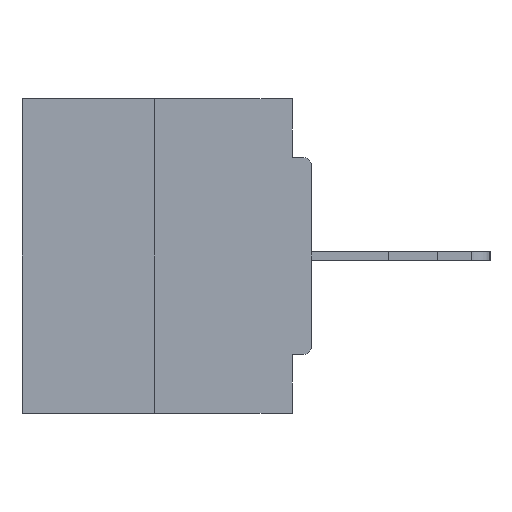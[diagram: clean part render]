
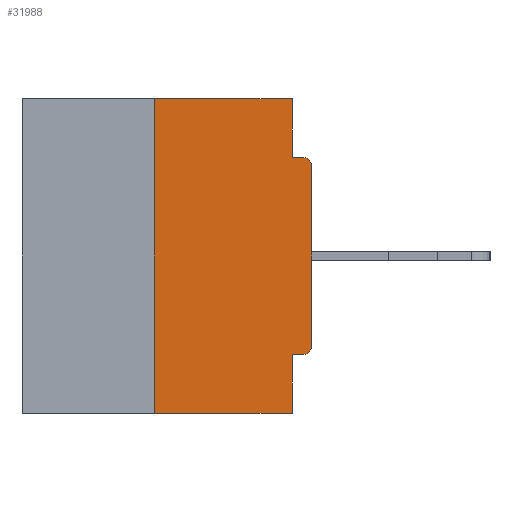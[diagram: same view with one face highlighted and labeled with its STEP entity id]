
A CAD part, left-side view. The second image highlights one B-rep face of the part: STEP entity #31988.
In plain terms, the highlighted planar face has unit normal (-1, 0, 0).
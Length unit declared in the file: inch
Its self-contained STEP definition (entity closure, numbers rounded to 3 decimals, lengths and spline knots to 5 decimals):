
#77 = CARTESIAN_POINT ( 'NONE',  ( 0., 0., -0.0935 ) ) ;
#569 = AXIS2_PLACEMENT_3D ( 'NONE', #17319, #38601, #14586 ) ;
#690 = VERTEX_POINT ( 'NONE', #12527 ) ;
#973 = VERTEX_POINT ( 'NONE', #18350 ) ;
#1141 = DIRECTION ( 'NONE',  ( -1., 0., 0. ) ) ;
#1912 = EDGE_LOOP ( 'NONE', ( #36719, #6356, #17836, #9807, #20751, #26262, #27287, #10193, #20718, #32546 ) ) ;
#2213 = LINE ( 'NONE', #35095, #6471 ) ;
#2317 = CARTESIAN_POINT ( 'NONE',  ( 0., 0.031, -0.5 ) ) ;
#2344 = EDGE_CURVE ( 'NONE', #28428, #690, #38097, .T. ) ;
#2489 = EDGE_CURVE ( 'NONE', #5081, #20839, #19757, .T. ) ;
#2567 = EDGE_CURVE ( 'NONE', #24842, #8759, #12766, .T. ) ;
#2583 = PLANE ( 'NONE',  #569 ) ;
#3424 = EDGE_CURVE ( 'NONE', #26230, #35803, #4994, .T. ) ;
#3914 = CARTESIAN_POINT ( 'NONE',  ( 0., 0.015, -0.3915 ) ) ;
#4805 = AXIS2_PLACEMENT_3D ( 'NONE', #9246, #12577, #23979 ) ;
#4994 = LINE ( 'NONE', #28396, #9011 ) ;
#5081 = VERTEX_POINT ( 'NONE', #28165 ) ;
#6230 = CARTESIAN_POINT ( 'NONE',  ( 0., 0.25, -0.5 ) ) ;
#6356 = ORIENTED_EDGE ( 'NONE', *, *, #19828, .F. ) ;
#6471 = VECTOR ( 'NONE', #8729, 39.37008 ) ;
#7024 = VECTOR ( 'NONE', #30851, 39.37008 ) ;
#8729 = DIRECTION ( 'NONE',  ( 0., 0., 1. ) ) ;
#8759 = VERTEX_POINT ( 'NONE', #32036 ) ;
#8926 = CARTESIAN_POINT ( 'NONE',  ( 0., 0., -0.4065 ) ) ;
#9011 = VECTOR ( 'NONE', #26002, 39.37008 ) ;
#9246 = CARTESIAN_POINT ( 'NONE',  ( 0., 0.015, -0.1085 ) ) ;
#9807 = ORIENTED_EDGE ( 'NONE', *, *, #31641, .F. ) ;
#10193 = ORIENTED_EDGE ( 'NONE', *, *, #2344, .T. ) ;
#10989 = VECTOR ( 'NONE', #30571, 39.37008 ) ;
#11890 = DIRECTION ( 'NONE',  ( 0., 0., -1. ) ) ;
#12142 = VECTOR ( 'NONE', #22022, 39.37008 ) ;
#12342 = CARTESIAN_POINT ( 'NONE',  ( 0., 0., -0.3915 ) ) ;
#12527 = CARTESIAN_POINT ( 'NONE',  ( 0., 0.015, -0.0935 ) ) ;
#12577 = DIRECTION ( 'NONE',  ( -1., 0., 0. ) ) ;
#12766 = LINE ( 'NONE', #21594, #38687 ) ;
#14586 = DIRECTION ( 'NONE',  ( 0., 0., -1. ) ) ;
#15889 = DIRECTION ( 'NONE',  ( 0., 0., -1. ) ) ;
#17319 = CARTESIAN_POINT ( 'NONE',  ( 0., 0.46, 0. ) ) ;
#17402 = CARTESIAN_POINT ( 'NONE',  ( 0., 0., -0.1085 ) ) ;
#17472 = EDGE_CURVE ( 'NONE', #973, #24842, #21799, .T. ) ;
#17836 = ORIENTED_EDGE ( 'NONE', *, *, #3424, .T. ) ;
#18350 = CARTESIAN_POINT ( 'NONE',  ( 0., 0.25, 0. ) ) ;
#19237 = CARTESIAN_POINT ( 'NONE',  ( 0., 0.46, 0. ) ) ;
#19389 = VECTOR ( 'NONE', #11890, 39.37008 ) ;
#19757 = CIRCLE ( 'NONE', #37392, 0.015 ) ;
#19828 = EDGE_CURVE ( 'NONE', #26230, #973, #2213, .T. ) ;
#20718 = ORIENTED_EDGE ( 'NONE', *, *, #27291, .F. ) ;
#20751 = ORIENTED_EDGE ( 'NONE', *, *, #22469, .F. ) ;
#20839 = VERTEX_POINT ( 'NONE', #12342 ) ;
#21468 = LINE ( 'NONE', #8926, #36106 ) ;
#21594 = CARTESIAN_POINT ( 'NONE',  ( 0., 0.031, 0. ) ) ;
#21799 = LINE ( 'NONE', #19237, #7024 ) ;
#22022 = DIRECTION ( 'NONE',  ( 0., 0., 1. ) ) ;
#22469 = EDGE_CURVE ( 'NONE', #5081, #28192, #21468, .T. ) ;
#23133 = CARTESIAN_POINT ( 'NONE',  ( 0., 0.031, 0. ) ) ;
#23979 = DIRECTION ( 'NONE',  ( 0., 0., -1. ) ) ;
#24267 = EDGE_CURVE ( 'NONE', #20839, #28428, #31272, .T. ) ;
#24842 = VERTEX_POINT ( 'NONE', #23133 ) ;
#26002 = DIRECTION ( 'NONE',  ( 0., -1., 0. ) ) ;
#26230 = VERTEX_POINT ( 'NONE', #6230 ) ;
#26262 = ORIENTED_EDGE ( 'NONE', *, *, #2489, .T. ) ;
#26564 = FACE_OUTER_BOUND ( 'NONE', #1912, .T. ) ;
#27186 = DIRECTION ( 'NONE',  ( 0., 1., 0. ) ) ;
#27287 = ORIENTED_EDGE ( 'NONE', *, *, #24267, .T. ) ;
#27291 = EDGE_CURVE ( 'NONE', #8759, #690, #33527, .T. ) ;
#28165 = CARTESIAN_POINT ( 'NONE',  ( 0., 0.015, -0.4065 ) ) ;
#28192 = VERTEX_POINT ( 'NONE', #33586 ) ;
#28396 = CARTESIAN_POINT ( 'NONE',  ( 0., 0.46, -0.5 ) ) ;
#28428 = VERTEX_POINT ( 'NONE', #17402 ) ;
#30571 = DIRECTION ( 'NONE',  ( 0., -1., 0. ) ) ;
#30851 = DIRECTION ( 'NONE',  ( 0., -1., 0. ) ) ;
#31272 = LINE ( 'NONE', #37003, #12142 ) ;
#31447 = DIRECTION ( 'NONE',  ( 0., 0., -1. ) ) ;
#31641 = EDGE_CURVE ( 'NONE', #28192, #35803, #38270, .T. ) ;
#31988 = ADVANCED_FACE ( 'NONE', ( #26564 ), #2583, .F. ) ;
#32036 = CARTESIAN_POINT ( 'NONE',  ( 0., 0.031, -0.0935 ) ) ;
#32546 = ORIENTED_EDGE ( 'NONE', *, *, #2567, .F. ) ;
#32919 = CARTESIAN_POINT ( 'NONE',  ( 0., 0.031, -0.5 ) ) ;
#33527 = LINE ( 'NONE', #77, #10989 ) ;
#33586 = CARTESIAN_POINT ( 'NONE',  ( 0., 0.031, -0.4065 ) ) ;
#35095 = CARTESIAN_POINT ( 'NONE',  ( 0., 0.25, 0. ) ) ;
#35803 = VERTEX_POINT ( 'NONE', #2317 ) ;
#36106 = VECTOR ( 'NONE', #27186, 39.37008 ) ;
#36719 = ORIENTED_EDGE ( 'NONE', *, *, #17472, .F. ) ;
#37003 = CARTESIAN_POINT ( 'NONE',  ( 0., 0., 0. ) ) ;
#37392 = AXIS2_PLACEMENT_3D ( 'NONE', #3914, #1141, #15889 ) ;
#38097 = CIRCLE ( 'NONE', #4805, 0.015 ) ;
#38270 = LINE ( 'NONE', #32919, #19389 ) ;
#38601 = DIRECTION ( 'NONE',  ( 1., 0., 0. ) ) ;
#38687 = VECTOR ( 'NONE', #31447, 39.37008 ) ;
